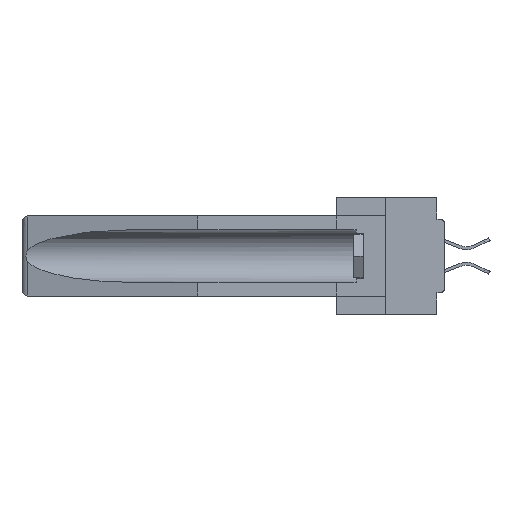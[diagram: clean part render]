
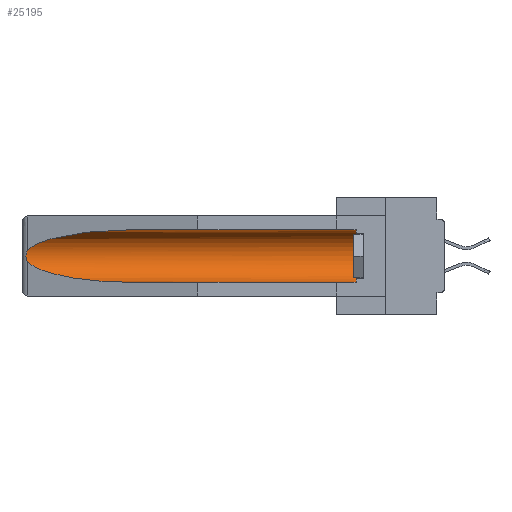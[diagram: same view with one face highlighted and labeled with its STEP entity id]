
A CAD part, left-side view. The second image highlights one B-rep face of the part: STEP entity #25195.
In plain terms, the highlighted cylindrical face has radius 2.857 mm (diameter 5.715 mm), a partial arc.
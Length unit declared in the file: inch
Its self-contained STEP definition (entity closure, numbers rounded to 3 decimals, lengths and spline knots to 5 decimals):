
#340 = EDGE_LOOP ( 'NONE', ( #3826, #39500, #37374, #5061, #6979, #12160 ) ) ;
#929 = CARTESIAN_POINT ( 'NONE',  ( 0.155, 1.07973, -0.284 ) ) ;
#1987 = CARTESIAN_POINT ( 'NONE',  ( 0.26537, 1.52718, -0.19328 ) ) ;
#2107 = CARTESIAN_POINT ( 'NONE',  ( 0.26537, 1.52718, -0.14972 ) ) ;
#2504 = CIRCLE ( 'NONE', #7337, 0.1125 ) ;
#3826 = ORIENTED_EDGE ( 'NONE', *, *, #4868, .T. ) ;
#4274 = AXIS2_PLACEMENT_3D ( 'NONE', #21848, #18821, #15509 ) ;
#4843 = CARTESIAN_POINT ( 'NONE',  ( 0.2673, 1.53269, -0.17917 ) ) ;
#4868 = EDGE_CURVE ( 'NONE', #8907, #28515, #15479, .T. ) ;
#5061 = ORIENTED_EDGE ( 'NONE', *, *, #23737, .F. ) ;
#5317 = CARTESIAN_POINT ( 'NONE',  ( 0.155, -0.30754, -0.059 ) ) ;
#6979 = ORIENTED_EDGE ( 'NONE', *, *, #27656, .T. ) ;
#7337 = AXIS2_PLACEMENT_3D ( 'NONE', #21910, #15291, #21767 ) ;
#8315 = DIRECTION ( 'NONE',  ( 0., 1., 0. ) ) ;
#8892 = FACE_OUTER_BOUND ( 'NONE', #340, .T. ) ;
#8907 = VERTEX_POINT ( 'NONE', #14011 ) ;
#11276 = CARTESIAN_POINT ( 'NONE',  ( 0.2673, 1.5327, -0.16383 ) ) ;
#12084 = VERTEX_POINT ( 'NONE', #20791 ) ;
#12160 = ORIENTED_EDGE ( 'NONE', *, *, #13365, .T. ) ;
#13221 = CARTESIAN_POINT ( 'NONE',  ( 0.155, 1.07973, -0.284 ) ) ;
#13365 = EDGE_CURVE ( 'NONE', #12084, #8907, #31401, .T. ) ;
#13987 = CYLINDRICAL_SURFACE ( 'NONE', #4274, 0.1125 ) ;
#14011 = CARTESIAN_POINT ( 'NONE',  ( 0.155, 1.07973, -0.059 ) ) ;
#14727 = CARTESIAN_POINT ( 'NONE',  ( 0.155, 0.126, -0.284 ) ) ;
#15291 = DIRECTION ( 'NONE',  ( 0., -1., 0. ) ) ;
#15479 =( BOUNDED_CURVE ( )  B_SPLINE_CURVE ( 3, ( #39086, #32351, #32912, #36107 ),
 .UNSPECIFIED., .F., .T. ) 
 B_SPLINE_CURVE_WITH_KNOTS ( ( 4, 4 ),
 ( 4.71239, 6.08839 ),
 .UNSPECIFIED. ) 
 CURVE ( )  GEOMETRIC_REPRESENTATION_ITEM ( )  RATIONAL_B_SPLINE_CURVE ( ( 1., 0.848, 0.848, 1. ) ) 
 REPRESENTATION_ITEM ( '' )  );
#15509 = DIRECTION ( 'NONE',  ( 0., 0., 1. ) ) ;
#17351 = EDGE_CURVE ( 'NONE', #22999, #31863, #20203, .T. ) ;
#17797 = CARTESIAN_POINT ( 'NONE',  ( 0.26654, 1.53092, -0.15636 ) ) ;
#18821 = DIRECTION ( 'NONE',  ( 0., 1., 0. ) ) ;
#20203 =( BOUNDED_CURVE ( )  B_SPLINE_CURVE ( 3, ( #40080, #27509, #37235, #929 ),
 .UNSPECIFIED., .F., .F. ) 
 B_SPLINE_CURVE_WITH_KNOTS ( ( 4, 4 ),
 ( 0.1948, 1.5708 ),
 .UNSPECIFIED. ) 
 CURVE ( )  GEOMETRIC_REPRESENTATION_ITEM ( )  RATIONAL_B_SPLINE_CURVE ( ( 1., 0.848, 0.848, 1. ) ) 
 REPRESENTATION_ITEM ( '' )  );
#20791 = CARTESIAN_POINT ( 'NONE',  ( 0.155, 0.126, -0.059 ) ) ;
#21767 = DIRECTION ( 'NONE',  ( 0., 0., 1. ) ) ;
#21848 = CARTESIAN_POINT ( 'NONE',  ( 0.155, -0.30754, -0.1715 ) ) ;
#21910 = CARTESIAN_POINT ( 'NONE',  ( 0.155, 0.126, -0.1715 ) ) ;
#22999 = VERTEX_POINT ( 'NONE', #1987 ) ;
#23737 = EDGE_CURVE ( 'NONE', #39696, #31863, #29868, .T. ) ;
#24389 = CARTESIAN_POINT ( 'NONE',  ( 0.2675, 1.53308, -0.17534 ) ) ;
#25195 = ADVANCED_FACE ( 'NONE', ( #8892 ), #13987, .F. ) ;
#27037 = B_SPLINE_CURVE_WITH_KNOTS ( 'NONE', 3,
 ( #2107, #31099, #17797, #11276, #40679, #24389, #4843, #41115, #37547, #37685 ),
 .UNSPECIFIED., .F., .F.,
 ( 4, 2, 2, 2, 4 ),
 ( 0., 0.00029, 0.00058, 0.00087, 0.00117 ),
 .UNSPECIFIED. ) ;
#27509 = CARTESIAN_POINT ( 'NONE',  ( 0.25451, 1.48313, -0.24835 ) ) ;
#27656 = EDGE_CURVE ( 'NONE', #39696, #12084, #2504, .T. ) ;
#28515 = VERTEX_POINT ( 'NONE', #42003 ) ;
#29155 = CARTESIAN_POINT ( 'NONE',  ( 0.155, -0.30754, -0.284 ) ) ;
#29868 = LINE ( 'NONE', #29155, #33425 ) ;
#31099 = CARTESIAN_POINT ( 'NONE',  ( 0.26597, 1.52961, -0.15275 ) ) ;
#31401 = LINE ( 'NONE', #5317, #38051 ) ;
#31863 = VERTEX_POINT ( 'NONE', #13221 ) ;
#32351 = CARTESIAN_POINT ( 'NONE',  ( 0.21114, 1.30732, -0.059 ) ) ;
#32428 = DIRECTION ( 'NONE',  ( 0., 1., 0. ) ) ;
#32912 = CARTESIAN_POINT ( 'NONE',  ( 0.25451, 1.48313, -0.09465 ) ) ;
#33425 = VECTOR ( 'NONE', #32428, 39.37008 ) ;
#36107 = CARTESIAN_POINT ( 'NONE',  ( 0.26537, 1.52718, -0.14972 ) ) ;
#36158 = EDGE_CURVE ( 'NONE', #28515, #22999, #27037, .T. ) ;
#37235 = CARTESIAN_POINT ( 'NONE',  ( 0.21114, 1.30732, -0.284 ) ) ;
#37374 = ORIENTED_EDGE ( 'NONE', *, *, #17351, .T. ) ;
#37547 = CARTESIAN_POINT ( 'NONE',  ( 0.26597, 1.5296, -0.19026 ) ) ;
#37685 = CARTESIAN_POINT ( 'NONE',  ( 0.26537, 1.52718, -0.19328 ) ) ;
#38051 = VECTOR ( 'NONE', #8315, 39.37008 ) ;
#39086 = CARTESIAN_POINT ( 'NONE',  ( 0.155, 1.07973, -0.059 ) ) ;
#39500 = ORIENTED_EDGE ( 'NONE', *, *, #36158, .T. ) ;
#39696 = VERTEX_POINT ( 'NONE', #14727 ) ;
#40080 = CARTESIAN_POINT ( 'NONE',  ( 0.26537, 1.52718, -0.19328 ) ) ;
#40679 = CARTESIAN_POINT ( 'NONE',  ( 0.2675, 1.53308, -0.16763 ) ) ;
#41115 = CARTESIAN_POINT ( 'NONE',  ( 0.26655, 1.53094, -0.18657 ) ) ;
#42003 = CARTESIAN_POINT ( 'NONE',  ( 0.26537, 1.52718, -0.14972 ) ) ;
